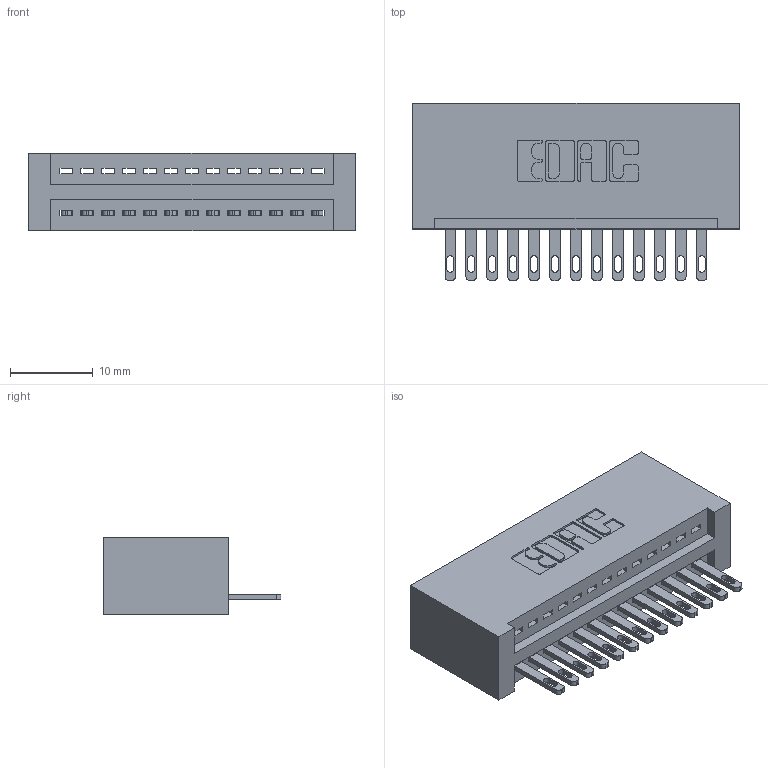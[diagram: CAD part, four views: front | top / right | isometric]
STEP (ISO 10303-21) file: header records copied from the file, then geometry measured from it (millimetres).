
FILE_DESCRIPTION (( 'STEP AP203' ), '1' );
FILE_NAME ('345-013-500-101.STEP', '2018-08-18T05:12:13', ( '' ), ( '' ), 'SwSTEP 2.0', 'SolidWorks 2016', '' );
FILE_SCHEMA (( 'CONFIG_CONTROL_DESIGN' ));
Length unit declared in the file: inch
Products named in the file (3): 345 Part_No Mounting Lugs; 345-292-001_345-293-100; 345-013-500-101
Assembly tree (14 placements, depth 2):
  345-013-500-101
    345 Part_No Mounting Lugs
    345-292-001_345-293-100  x13
Bounding box: 39.62 x 21.51 x 9.4 mm (x, y, z)
Volume: 4118.4 mm3; surface area: 5298.1 mm2
Topology: 14 solids, 14 shells, 820 faces, 2501 edges, 1666 vertices
Faces by surface type: plane 518, cylinder 302
Entity records: 13341 total; most frequent: CARTESIAN_POINT 2319, ORIENTED_EDGE 2266, DIRECTION 2063, EDGE_CURVE 1133, VECTOR 953, LINE 953, VERTEX_POINT 754, AXIS2_PLACEMENT_3D 555
